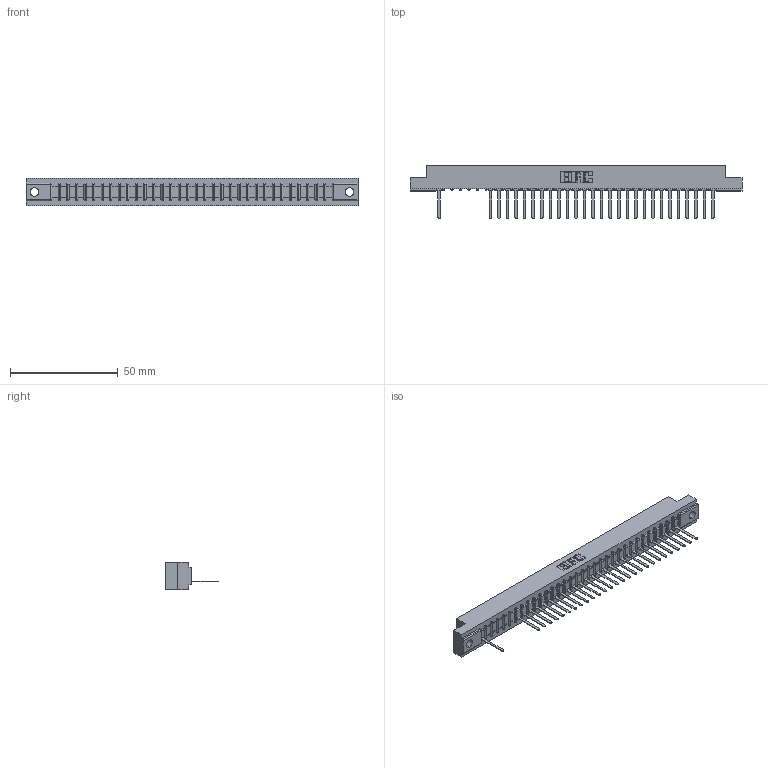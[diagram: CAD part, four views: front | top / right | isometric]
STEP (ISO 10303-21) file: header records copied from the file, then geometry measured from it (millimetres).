
FILE_DESCRIPTION (( 'STEP AP203' ), '1' );
FILE_NAME ('357-033-541-104.STEP', '2018-08-10T01:29:21', ( '' ), ( '' ), 'SwSTEP 2.0', 'SolidWorks 2016', '' );
FILE_SCHEMA (( 'CONFIG_CONTROL_DESIGN' ));
Length unit declared in the file: inch
Products named in the file (3): 307 Part_.156 Dia Mounting Holes; 307-290-002_541; 357-033-541-104
Assembly tree (29 placements, depth 2):
  357-033-541-104
    307 Part_.156 Dia Mounting Holes
    307-290-002_541  x28
Bounding box: 153.77 x 24.59 x 12.7 mm (x, y, z)
Volume: 16216.8 mm3; surface area: 19610.9 mm2
Topology: 29 solids, 29 shells, 2338 faces, 7175 edges, 4690 vertices
Faces by surface type: plane 1404, cylinder 866, sphere 68
Entity records: 30376 total; most frequent: CARTESIAN_POINT 5149, ORIENTED_EDGE 5142, DIRECTION 4993, EDGE_CURVE 2571, VECTOR 1973, LINE 1973, VERTEX_POINT 1666, AXIS2_PLACEMENT_3D 1510
